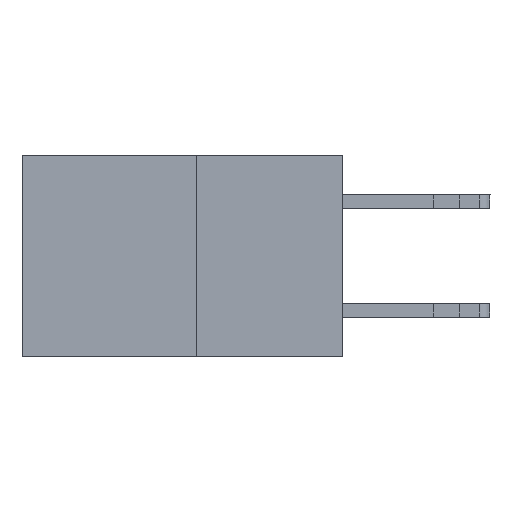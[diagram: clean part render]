
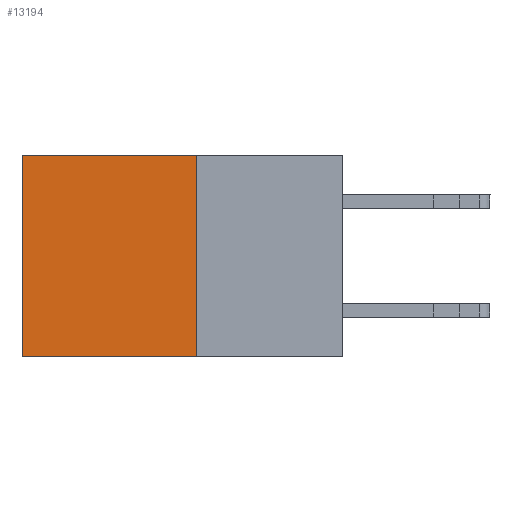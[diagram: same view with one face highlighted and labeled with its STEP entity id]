
A CAD part, left-side view. The second image highlights one B-rep face of the part: STEP entity #13194.
In plain terms, the highlighted planar face has unit normal (-1, 0, 0).
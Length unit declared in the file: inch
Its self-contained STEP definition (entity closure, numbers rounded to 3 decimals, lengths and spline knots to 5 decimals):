
#873 = PLANE ( 'NONE',  #2518 ) ;
#1158 = EDGE_CURVE ( 'NONE', #15018, #6765, #2186, .T. ) ;
#1636 = CARTESIAN_POINT ( 'NONE',  ( 0.277, 0.27, -0.37 ) ) ;
#2022 = VERTEX_POINT ( 'NONE', #2335 ) ;
#2186 = LINE ( 'NONE', #13069, #11882 ) ;
#2202 = CARTESIAN_POINT ( 'NONE',  ( 0.277, 0.27, -0.37 ) ) ;
#2303 = LINE ( 'NONE', #1636, #2737 ) ;
#2335 = CARTESIAN_POINT ( 'NONE',  ( 0.277, 0.27, -0.37 ) ) ;
#2412 = VERTEX_POINT ( 'NONE', #11466 ) ;
#2464 = EDGE_LOOP ( 'NONE', ( #12369, #10322, #8921, #9719 ) ) ;
#2518 = AXIS2_PLACEMENT_3D ( 'NONE', #2202, #11417, #3537 ) ;
#2737 = VECTOR ( 'NONE', #8223, 39.37008 ) ;
#2959 = CARTESIAN_POINT ( 'NONE',  ( 0.277, 0.59, 0. ) ) ;
#3378 = DIRECTION ( 'NONE',  ( 0., 1., 0. ) ) ;
#3537 = DIRECTION ( 'NONE',  ( 0., 0., -1. ) ) ;
#3860 = LINE ( 'NONE', #15752, #10407 ) ;
#6569 = CARTESIAN_POINT ( 'NONE',  ( 0.277, 0.59, -0.37 ) ) ;
#6765 = VERTEX_POINT ( 'NONE', #6569 ) ;
#7268 = EDGE_CURVE ( 'NONE', #2412, #15018, #3860, .T. ) ;
#7311 = CARTESIAN_POINT ( 'NONE',  ( 0.277, 0.27, -0.37 ) ) ;
#8223 = DIRECTION ( 'NONE',  ( 0., 0., -1. ) ) ;
#8921 = ORIENTED_EDGE ( 'NONE', *, *, #15024, .F. ) ;
#9441 = VECTOR ( 'NONE', #3378, 39.37008 ) ;
#9719 = ORIENTED_EDGE ( 'NONE', *, *, #7268, .T. ) ;
#10097 = DIRECTION ( 'NONE',  ( 0., 0., -1. ) ) ;
#10247 = LINE ( 'NONE', #7311, #9441 ) ;
#10322 = ORIENTED_EDGE ( 'NONE', *, *, #16379, .F. ) ;
#10407 = VECTOR ( 'NONE', #14486, 39.37008 ) ;
#11417 = DIRECTION ( 'NONE',  ( 1., 0., 0. ) ) ;
#11466 = CARTESIAN_POINT ( 'NONE',  ( 0.277, 0.27, 0. ) ) ;
#11882 = VECTOR ( 'NONE', #10097, 39.37008 ) ;
#12369 = ORIENTED_EDGE ( 'NONE', *, *, #1158, .T. ) ;
#13069 = CARTESIAN_POINT ( 'NONE',  ( 0.277, 0.59, -0.37 ) ) ;
#13194 = ADVANCED_FACE ( 'NONE', ( #14876 ), #873, .F. ) ;
#14486 = DIRECTION ( 'NONE',  ( 0., 1., 0. ) ) ;
#14876 = FACE_OUTER_BOUND ( 'NONE', #2464, .T. ) ;
#15018 = VERTEX_POINT ( 'NONE', #2959 ) ;
#15024 = EDGE_CURVE ( 'NONE', #2412, #2022, #2303, .T. ) ;
#15752 = CARTESIAN_POINT ( 'NONE',  ( 0.277, 0.27, 0. ) ) ;
#16379 = EDGE_CURVE ( 'NONE', #2022, #6765, #10247, .T. ) ;
